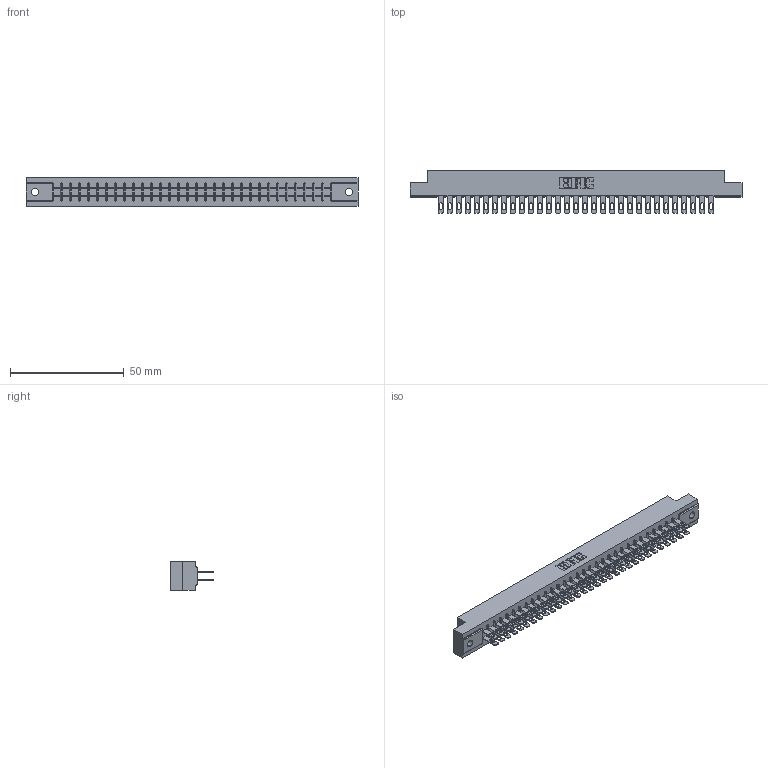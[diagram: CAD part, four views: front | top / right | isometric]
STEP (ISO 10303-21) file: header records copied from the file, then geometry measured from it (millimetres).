
FILE_DESCRIPTION (( 'STEP AP203' ), '1' );
FILE_NAME ('355-062-500-502.STEP', '2019-09-12T14:14:04', ( '' ), ( '' ), 'SwSTEP 2.0', 'SolidWorks 2016', '' );
FILE_SCHEMA (( 'CONFIG_CONTROL_DESIGN' ));
Length unit declared in the file: inch
Products named in the file (3): 305-290-001_500; 355-062-500-502; 305 Part_.128 Dia
Assembly tree (63 placements, depth 2):
  355-062-500-502
    305 Part_.128 Dia
    305-290-001_500  x62
Bounding box: 145.85 x 18.85 x 12.7 mm (x, y, z)
Volume: 14874.6 mm3; surface area: 20303.2 mm2
Topology: 63 solids, 63 shells, 3216 faces, 9213 edges, 5974 vertices
Faces by surface type: plane 1804, cylinder 1288, sphere 124
Entity records: 34928 total; most frequent: CARTESIAN_POINT 5779, ORIENTED_EDGE 5734, DIRECTION 5601, EDGE_CURVE 2867, VECTOR 2305, LINE 2305, VERTEX_POINT 1826, AXIS2_PLACEMENT_3D 1648
